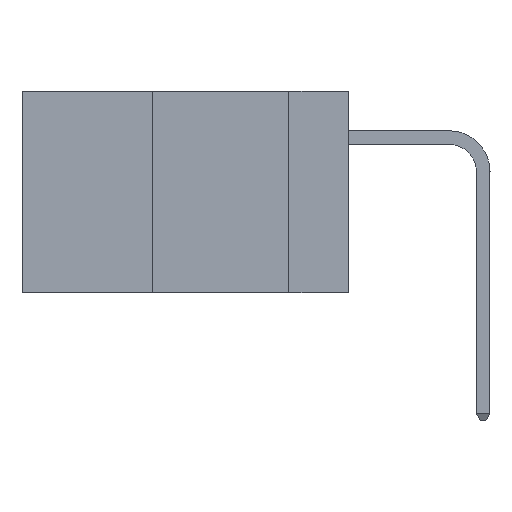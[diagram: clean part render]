
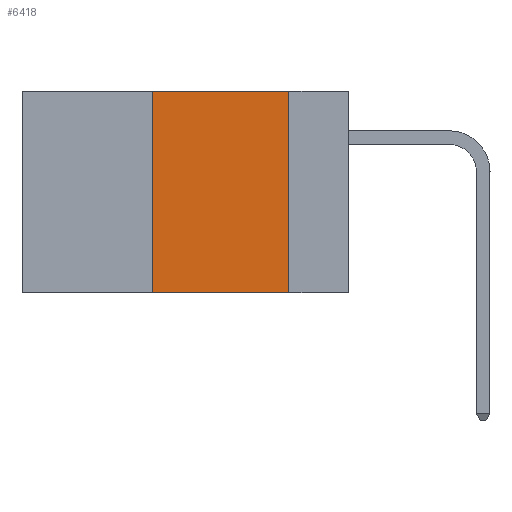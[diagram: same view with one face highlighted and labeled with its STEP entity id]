
A CAD part, left-side view. The second image highlights one B-rep face of the part: STEP entity #6418.
In plain terms, the highlighted planar face has unit normal (-1, 0, 0).
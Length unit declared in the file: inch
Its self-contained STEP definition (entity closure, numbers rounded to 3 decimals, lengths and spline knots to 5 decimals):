
#451 = VERTEX_POINT ( 'NONE', #1176 ) ;
#495 = EDGE_CURVE ( 'NONE', #451, #12469, #2746, .T. ) ;
#1176 = CARTESIAN_POINT ( 'NONE',  ( 0., 0.36, 0. ) ) ;
#1884 = DIRECTION ( 'NONE',  ( 0., -1., 0. ) ) ;
#2331 = EDGE_CURVE ( 'NONE', #5227, #451, #4696, .T. ) ;
#2524 = ORIENTED_EDGE ( 'NONE', *, *, #2331, .F. ) ;
#2746 = LINE ( 'NONE', #4373, #11022 ) ;
#2919 = CARTESIAN_POINT ( 'NONE',  ( 0., 0.6, 0. ) ) ;
#3792 = DIRECTION ( 'NONE',  ( 0., 0., 1. ) ) ;
#3866 = FACE_OUTER_BOUND ( 'NONE', #4021, .T. ) ;
#4021 = EDGE_LOOP ( 'NONE', ( #9483, #6685, #2524, #7343 ) ) ;
#4195 = AXIS2_PLACEMENT_3D ( 'NONE', #2919, #12366, #11403 ) ;
#4373 = CARTESIAN_POINT ( 'NONE',  ( 0., 0.6, 0. ) ) ;
#4534 = EDGE_CURVE ( 'NONE', #12469, #9827, #12116, .T. ) ;
#4657 = EDGE_CURVE ( 'NONE', #5227, #9827, #8523, .T. ) ;
#4696 = LINE ( 'NONE', #5690, #12114 ) ;
#5227 = VERTEX_POINT ( 'NONE', #7721 ) ;
#5690 = CARTESIAN_POINT ( 'NONE',  ( 0., 0.36, 0. ) ) ;
#6017 = VECTOR ( 'NONE', #1884, 39.37008 ) ;
#6418 = ADVANCED_FACE ( 'NONE', ( #3866 ), #11582, .F. ) ;
#6685 = ORIENTED_EDGE ( 'NONE', *, *, #495, .F. ) ;
#7343 = ORIENTED_EDGE ( 'NONE', *, *, #4657, .T. ) ;
#7721 = CARTESIAN_POINT ( 'NONE',  ( 0., 0.36, -0.37 ) ) ;
#8523 = LINE ( 'NONE', #10468, #6017 ) ;
#9483 = ORIENTED_EDGE ( 'NONE', *, *, #4534, .F. ) ;
#9827 = VERTEX_POINT ( 'NONE', #12404 ) ;
#10143 = CARTESIAN_POINT ( 'NONE',  ( 0., 0.11, 0. ) ) ;
#10468 = CARTESIAN_POINT ( 'NONE',  ( 0., 0.6, -0.37 ) ) ;
#11022 = VECTOR ( 'NONE', #11343, 39.37008 ) ;
#11343 = DIRECTION ( 'NONE',  ( 0., -1., 0. ) ) ;
#11403 = DIRECTION ( 'NONE',  ( 0., 0., -1. ) ) ;
#11582 = PLANE ( 'NONE',  #4195 ) ;
#11652 = CARTESIAN_POINT ( 'NONE',  ( 0., 0.11, 0. ) ) ;
#12114 = VECTOR ( 'NONE', #3792, 39.37008 ) ;
#12116 = LINE ( 'NONE', #10143, #12307 ) ;
#12178 = DIRECTION ( 'NONE',  ( 0., 0., -1. ) ) ;
#12307 = VECTOR ( 'NONE', #12178, 39.37008 ) ;
#12366 = DIRECTION ( 'NONE',  ( 1., 0., 0. ) ) ;
#12404 = CARTESIAN_POINT ( 'NONE',  ( 0., 0.11, -0.37 ) ) ;
#12469 = VERTEX_POINT ( 'NONE', #11652 ) ;
